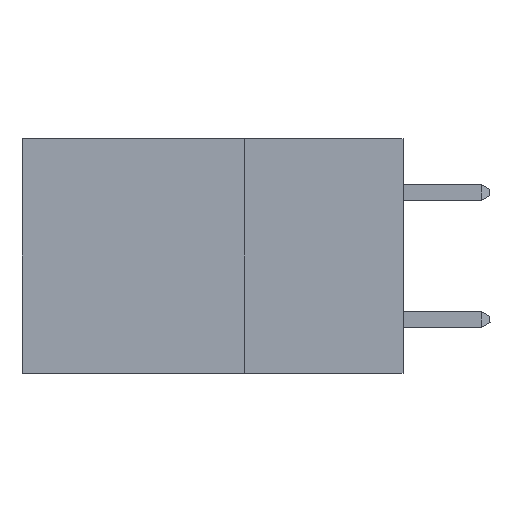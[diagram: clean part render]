
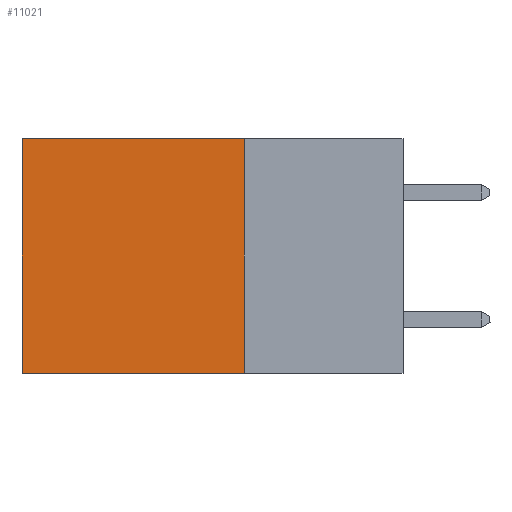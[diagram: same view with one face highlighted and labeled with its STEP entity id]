
A CAD part, left-side view. The second image highlights one B-rep face of the part: STEP entity #11021.
In plain terms, the highlighted planar face has unit normal (-1, 0, 0).
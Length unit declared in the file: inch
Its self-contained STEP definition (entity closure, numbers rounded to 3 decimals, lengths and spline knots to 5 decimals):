
#76 = DIRECTION ( 'NONE',  ( 0., 1., 0. ) ) ;
#631 = EDGE_CURVE ( 'NONE', #14473, #14326, #9453, .T. ) ;
#778 = VECTOR ( 'NONE', #29998, 39.37008 ) ;
#6783 = ORIENTED_EDGE ( 'NONE', *, *, #17695, .T. ) ;
#7296 = CARTESIAN_POINT ( 'NONE',  ( 0.2875, 0.25, -0.37 ) ) ;
#7470 = VECTOR ( 'NONE', #30789, 39.37008 ) ;
#7651 = LINE ( 'NONE', #40606, #32528 ) ;
#7663 = CARTESIAN_POINT ( 'NONE',  ( 0.2875, 0.25, 0. ) ) ;
#9121 = EDGE_CURVE ( 'NONE', #12632, #14326, #24809, .T. ) ;
#9453 = LINE ( 'NONE', #7296, #778 ) ;
#9947 = EDGE_LOOP ( 'NONE', ( #26359, #29947, #40136, #6783 ) ) ;
#10431 = FACE_OUTER_BOUND ( 'NONE', #9947, .T. ) ;
#10940 = PLANE ( 'NONE',  #24138 ) ;
#11021 = ADVANCED_FACE ( 'NONE', ( #10431 ), #10940, .F. ) ;
#11640 = CARTESIAN_POINT ( 'NONE',  ( 0.2875, 0.25, -0.37 ) ) ;
#11820 = VECTOR ( 'NONE', #76, 39.37008 ) ;
#12632 = VERTEX_POINT ( 'NONE', #21641 ) ;
#14172 = VERTEX_POINT ( 'NONE', #29085 ) ;
#14220 = CARTESIAN_POINT ( 'NONE',  ( 0.2875, 0.6, -0.37 ) ) ;
#14232 = DIRECTION ( 'NONE',  ( 1., 0., 0. ) ) ;
#14326 = VERTEX_POINT ( 'NONE', #14220 ) ;
#14473 = VERTEX_POINT ( 'NONE', #11640 ) ;
#17695 = EDGE_CURVE ( 'NONE', #14172, #12632, #20522, .T. ) ;
#20522 = LINE ( 'NONE', #38974, #11820 ) ;
#21641 = CARTESIAN_POINT ( 'NONE',  ( 0.2875, 0.6, 0. ) ) ;
#24138 = AXIS2_PLACEMENT_3D ( 'NONE', #7663, #14232, #36851 ) ;
#24809 = LINE ( 'NONE', #27513, #7470 ) ;
#26359 = ORIENTED_EDGE ( 'NONE', *, *, #9121, .T. ) ;
#27513 = CARTESIAN_POINT ( 'NONE',  ( 0.2875, 0.6, 0. ) ) ;
#29085 = CARTESIAN_POINT ( 'NONE',  ( 0.2875, 0.25, 0. ) ) ;
#29947 = ORIENTED_EDGE ( 'NONE', *, *, #631, .F. ) ;
#29998 = DIRECTION ( 'NONE',  ( 0., 1., 0. ) ) ;
#30789 = DIRECTION ( 'NONE',  ( 0., 0., -1. ) ) ;
#32528 = VECTOR ( 'NONE', #40744, 39.37008 ) ;
#36851 = DIRECTION ( 'NONE',  ( 0., 0., -1. ) ) ;
#38974 = CARTESIAN_POINT ( 'NONE',  ( 0.2875, 0.25, 0. ) ) ;
#40136 = ORIENTED_EDGE ( 'NONE', *, *, #41385, .F. ) ;
#40606 = CARTESIAN_POINT ( 'NONE',  ( 0.2875, 0.25, 0. ) ) ;
#40744 = DIRECTION ( 'NONE',  ( 0., 0., -1. ) ) ;
#41385 = EDGE_CURVE ( 'NONE', #14172, #14473, #7651, .T. ) ;
